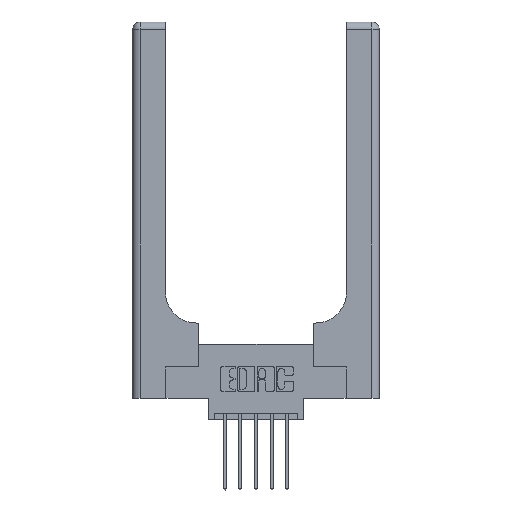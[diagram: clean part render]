
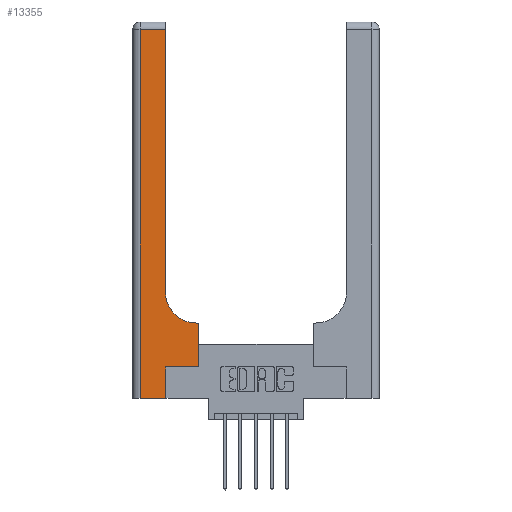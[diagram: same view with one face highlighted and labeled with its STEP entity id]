
A CAD part, top view. The second image highlights one B-rep face of the part: STEP entity #13355.
In plain terms, the highlighted planar face has unit normal (0, 0, 1).
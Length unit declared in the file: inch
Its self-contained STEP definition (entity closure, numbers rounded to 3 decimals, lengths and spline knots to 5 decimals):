
#2 = VECTOR ( 'NONE', #12881, 39.37008 ) ;
#50 = CARTESIAN_POINT ( 'NONE',  ( 0.528, 0.6, 0.37 ) ) ;
#75 = VECTOR ( 'NONE', #12997, 39.37008 ) ;
#276 = VECTOR ( 'NONE', #1674, 39.37008 ) ;
#398 = ORIENTED_EDGE ( 'NONE', *, *, #4802, .T. ) ;
#611 = CARTESIAN_POINT ( 'NONE',  ( 0., 2.94, 0.37 ) ) ;
#655 = LINE ( 'NONE', #7695, #2 ) ;
#656 = EDGE_CURVE ( 'NONE', #7561, #8321, #7871, .T. ) ;
#726 = CARTESIAN_POINT ( 'NONE',  ( 0.06, 2.94, 0.37 ) ) ;
#803 = LINE ( 'NONE', #11287, #11643 ) ;
#1088 = DIRECTION ( 'NONE',  ( 0., 0., -1. ) ) ;
#1509 = VERTEX_POINT ( 'NONE', #8513 ) ;
#1528 = EDGE_LOOP ( 'NONE', ( #398, #4205, #4874, #8019, #3371, #9315, #4706, #2231, #5709 ) ) ;
#1674 = DIRECTION ( 'NONE',  ( -1., 0., 0. ) ) ;
#1677 = EDGE_CURVE ( 'NONE', #8321, #2537, #10909, .T. ) ;
#2011 = CARTESIAN_POINT ( 'NONE',  ( 0.265, 0., 0.37 ) ) ;
#2086 = VERTEX_POINT ( 'NONE', #11662 ) ;
#2231 = ORIENTED_EDGE ( 'NONE', *, *, #2562, .T. ) ;
#2296 = DIRECTION ( 'NONE',  ( 0., 0., -1. ) ) ;
#2537 = VERTEX_POINT ( 'NONE', #50 ) ;
#2562 = EDGE_CURVE ( 'NONE', #2537, #4772, #12220, .T. ) ;
#2890 = DIRECTION ( 'NONE',  ( 1., 0., 0. ) ) ;
#3064 = DIRECTION ( 'NONE',  ( 0., 1., 0. ) ) ;
#3371 = ORIENTED_EDGE ( 'NONE', *, *, #12627, .T. ) ;
#3627 = AXIS2_PLACEMENT_3D ( 'NONE', #7433, #1088, #8467 ) ;
#3677 = CARTESIAN_POINT ( 'NONE',  ( 0.265, 0.25, 0.37 ) ) ;
#3834 = CARTESIAN_POINT ( 'NONE',  ( 0.06, 3., 0.37 ) ) ;
#4101 = CIRCLE ( 'NONE', #3627, 0.25 ) ;
#4205 = ORIENTED_EDGE ( 'NONE', *, *, #8745, .T. ) ;
#4613 = CARTESIAN_POINT ( 'NONE',  ( 0.528, 0.25, 0.37 ) ) ;
#4706 = ORIENTED_EDGE ( 'NONE', *, *, #1677, .T. ) ;
#4756 = DIRECTION ( 'NONE',  ( 1., 0., 0. ) ) ;
#4772 = VERTEX_POINT ( 'NONE', #8648 ) ;
#4802 = EDGE_CURVE ( 'NONE', #2086, #9084, #655, .T. ) ;
#4874 = ORIENTED_EDGE ( 'NONE', *, *, #10486, .T. ) ;
#5373 = CARTESIAN_POINT ( 'NONE',  ( 0.26, 0.6, 0.37 ) ) ;
#5476 = VERTEX_POINT ( 'NONE', #726 ) ;
#5522 = EDGE_CURVE ( 'NONE', #1509, #11352, #803, .T. ) ;
#5698 = EDGE_CURVE ( 'NONE', #4772, #2086, #4101, .T. ) ;
#5709 = ORIENTED_EDGE ( 'NONE', *, *, #5698, .T. ) ;
#5914 = LINE ( 'NONE', #611, #276 ) ;
#6043 = LINE ( 'NONE', #2011, #10600 ) ;
#6383 = DIRECTION ( 'NONE',  ( -1., 0., 0. ) ) ;
#6388 = AXIS2_PLACEMENT_3D ( 'NONE', #9618, #2296, #9666 ) ;
#6433 = VECTOR ( 'NONE', #13286, 39.37008 ) ;
#6517 = PLANE ( 'NONE',  #6388 ) ;
#7433 = CARTESIAN_POINT ( 'NONE',  ( 0.51, 0.85, 0.37 ) ) ;
#7561 = VERTEX_POINT ( 'NONE', #8518 ) ;
#7695 = CARTESIAN_POINT ( 'NONE',  ( 0.26, 3., 0.37 ) ) ;
#7871 = LINE ( 'NONE', #3677, #13080 ) ;
#8019 = ORIENTED_EDGE ( 'NONE', *, *, #5522, .T. ) ;
#8321 = VERTEX_POINT ( 'NONE', #10403 ) ;
#8328 = FACE_OUTER_BOUND ( 'NONE', #1528, .T. ) ;
#8467 = DIRECTION ( 'NONE',  ( 1., 0., 0. ) ) ;
#8513 = CARTESIAN_POINT ( 'NONE',  ( 0.06, 0., 0.37 ) ) ;
#8518 = CARTESIAN_POINT ( 'NONE',  ( 0.265, 0.25, 0.37 ) ) ;
#8648 = CARTESIAN_POINT ( 'NONE',  ( 0.51, 0.6, 0.37 ) ) ;
#8745 = EDGE_CURVE ( 'NONE', #9084, #5476, #5914, .T. ) ;
#9084 = VERTEX_POINT ( 'NONE', #9538 ) ;
#9210 = LINE ( 'NONE', #3834, #6433 ) ;
#9315 = ORIENTED_EDGE ( 'NONE', *, *, #656, .T. ) ;
#9538 = CARTESIAN_POINT ( 'NONE',  ( 0.26, 2.94, 0.37 ) ) ;
#9618 = CARTESIAN_POINT ( 'NONE',  ( 0., 3., 0.37 ) ) ;
#9666 = DIRECTION ( 'NONE',  ( -1., 0., 0. ) ) ;
#10087 = VECTOR ( 'NONE', #6383, 39.37008 ) ;
#10403 = CARTESIAN_POINT ( 'NONE',  ( 0.528, 0.25, 0.37 ) ) ;
#10486 = EDGE_CURVE ( 'NONE', #5476, #1509, #9210, .T. ) ;
#10600 = VECTOR ( 'NONE', #3064, 39.37008 ) ;
#10909 = LINE ( 'NONE', #4613, #75 ) ;
#11174 = CARTESIAN_POINT ( 'NONE',  ( 0.265, 0., 0.37 ) ) ;
#11287 = CARTESIAN_POINT ( 'NONE',  ( 0., 0., 0.37 ) ) ;
#11352 = VERTEX_POINT ( 'NONE', #11174 ) ;
#11643 = VECTOR ( 'NONE', #2890, 39.37008 ) ;
#11662 = CARTESIAN_POINT ( 'NONE',  ( 0.26, 0.85, 0.37 ) ) ;
#12220 = LINE ( 'NONE', #5373, #10087 ) ;
#12627 = EDGE_CURVE ( 'NONE', #11352, #7561, #6043, .T. ) ;
#12881 = DIRECTION ( 'NONE',  ( 0., 1., 0. ) ) ;
#12997 = DIRECTION ( 'NONE',  ( 0., 1., 0. ) ) ;
#13080 = VECTOR ( 'NONE', #4756, 39.37008 ) ;
#13286 = DIRECTION ( 'NONE',  ( 0., -1., 0. ) ) ;
#13355 = ADVANCED_FACE ( 'NONE', ( #8328 ), #6517, .F. ) ;
